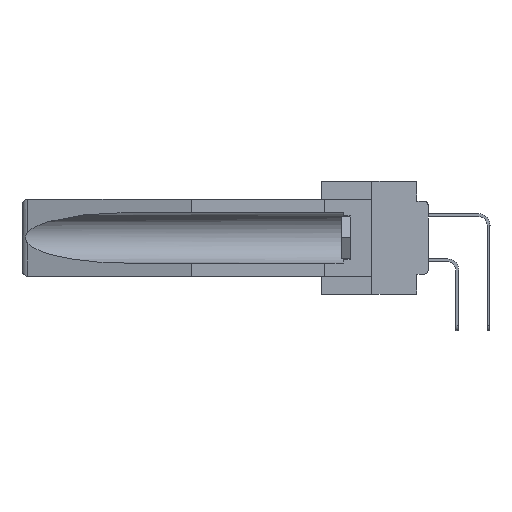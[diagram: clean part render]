
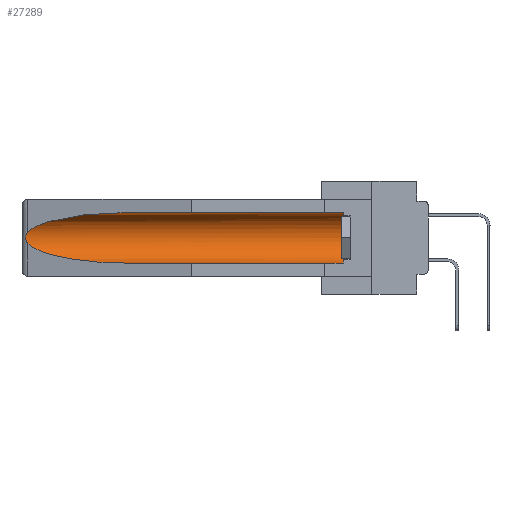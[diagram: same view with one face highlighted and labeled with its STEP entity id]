
A CAD part, left-side view. The second image highlights one B-rep face of the part: STEP entity #27289.
In plain terms, the highlighted cylindrical face has radius 2.857 mm (diameter 5.715 mm), a partial arc.
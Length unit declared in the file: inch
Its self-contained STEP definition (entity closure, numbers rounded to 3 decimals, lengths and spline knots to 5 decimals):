
#214 = VECTOR ( 'NONE', #16358, 39.37008 ) ;
#220 = EDGE_CURVE ( 'NONE', #14989, #16163, #27075, .T. ) ;
#622 = LINE ( 'NONE', #17591, #22958 ) ;
#1041 = CARTESIAN_POINT ( 'NONE',  ( 0.2675, 1.53308, -0.17534 ) ) ;
#2918 = VERTEX_POINT ( 'NONE', #24514 ) ;
#2966 = CARTESIAN_POINT ( 'NONE',  ( 0.25451, 1.48313, -0.24835 ) ) ;
#3231 = EDGE_LOOP ( 'NONE', ( #13772, #20489, #29603, #16007, #25801, #6944 ) ) ;
#3572 = CARTESIAN_POINT ( 'NONE',  ( 0.26537, 1.52718, -0.14972 ) ) ;
#3773 = CARTESIAN_POINT ( 'NONE',  ( 0.21114, 1.30732, -0.059 ) ) ;
#5889 = CARTESIAN_POINT ( 'NONE',  ( 0.26537, 1.52718, -0.19328 ) ) ;
#6092 = CARTESIAN_POINT ( 'NONE',  ( 0.2673, 1.53269, -0.17917 ) ) ;
#6944 = ORIENTED_EDGE ( 'NONE', *, *, #20232, .T. ) ;
#7067 = CARTESIAN_POINT ( 'NONE',  ( 0.155, -0.30754, -0.1715 ) ) ;
#7306 = DIRECTION ( 'NONE',  ( 0., 0., 1. ) ) ;
#7380 = DIRECTION ( 'NONE',  ( 0., 1., 0. ) ) ;
#8612 = VERTEX_POINT ( 'NONE', #22901 ) ;
#8885 = EDGE_CURVE ( 'NONE', #26330, #2918, #29092, .T. ) ;
#10323 = CARTESIAN_POINT ( 'NONE',  ( 0.26537, 1.52718, -0.14972 ) ) ;
#11713 = EDGE_CURVE ( 'NONE', #14989, #24614, #28343, .T. ) ;
#12687 = CARTESIAN_POINT ( 'NONE',  ( 0.155, 0.126, -0.284 ) ) ;
#13161 = CARTESIAN_POINT ( 'NONE',  ( 0.26654, 1.53092, -0.15636 ) ) ;
#13772 = ORIENTED_EDGE ( 'NONE', *, *, #15866, .T. ) ;
#13786 = CYLINDRICAL_SURFACE ( 'NONE', #28891, 0.1125 ) ;
#14078 = CARTESIAN_POINT ( 'NONE',  ( 0.155, 1.07973, -0.284 ) ) ;
#14661 = CARTESIAN_POINT ( 'NONE',  ( 0.155, 0.126, -0.1715 ) ) ;
#14989 = VERTEX_POINT ( 'NONE', #12687 ) ;
#15505 = CARTESIAN_POINT ( 'NONE',  ( 0.26537, 1.52718, -0.19328 ) ) ;
#15866 = EDGE_CURVE ( 'NONE', #8612, #26330, #23485, .T. ) ;
#16007 = ORIENTED_EDGE ( 'NONE', *, *, #220, .F. ) ;
#16163 = VERTEX_POINT ( 'NONE', #14078 ) ;
#16358 = DIRECTION ( 'NONE',  ( 0., 1., 0. ) ) ;
#16474 = CARTESIAN_POINT ( 'NONE',  ( 0.155, -0.30754, -0.284 ) ) ;
#16822 = DIRECTION ( 'NONE',  ( 0., -1., 0. ) ) ;
#17359 = CARTESIAN_POINT ( 'NONE',  ( 0.155, 1.07973, -0.284 ) ) ;
#17591 = CARTESIAN_POINT ( 'NONE',  ( 0.155, -0.30754, -0.059 ) ) ;
#17766 = CARTESIAN_POINT ( 'NONE',  ( 0.2673, 1.5327, -0.16383 ) ) ;
#17868 = CARTESIAN_POINT ( 'NONE',  ( 0.26655, 1.53094, -0.18657 ) ) ;
#18258 = CARTESIAN_POINT ( 'NONE',  ( 0.155, 0.126, -0.059 ) ) ;
#19763 = CARTESIAN_POINT ( 'NONE',  ( 0.26537, 1.52718, -0.14972 ) ) ;
#19903 = FACE_OUTER_BOUND ( 'NONE', #3231, .T. ) ;
#20130 = DIRECTION ( 'NONE',  ( 0., 1., 0. ) ) ;
#20232 = EDGE_CURVE ( 'NONE', #24614, #8612, #622, .T. ) ;
#20401 = CARTESIAN_POINT ( 'NONE',  ( 0.26597, 1.52961, -0.15275 ) ) ;
#20489 = ORIENTED_EDGE ( 'NONE', *, *, #8885, .T. ) ;
#20605 = CARTESIAN_POINT ( 'NONE',  ( 0.2675, 1.53308, -0.16763 ) ) ;
#20769 =( BOUNDED_CURVE ( )  B_SPLINE_CURVE ( 3, ( #15505, #2966, #22012, #17359 ),
 .UNSPECIFIED., .F., .F. ) 
 B_SPLINE_CURVE_WITH_KNOTS ( ( 4, 4 ),
 ( 0.1948, 1.5708 ),
 .UNSPECIFIED. ) 
 CURVE ( )  GEOMETRIC_REPRESENTATION_ITEM ( )  RATIONAL_B_SPLINE_CURVE ( ( 1., 0.848, 0.848, 1. ) ) 
 REPRESENTATION_ITEM ( '' )  );
#21565 = DIRECTION ( 'NONE',  ( 0., 0., 1. ) ) ;
#21851 = AXIS2_PLACEMENT_3D ( 'NONE', #14661, #16822, #7306 ) ;
#22012 = CARTESIAN_POINT ( 'NONE',  ( 0.21114, 1.30732, -0.284 ) ) ;
#22901 = CARTESIAN_POINT ( 'NONE',  ( 0.155, 1.07973, -0.059 ) ) ;
#22958 = VECTOR ( 'NONE', #20130, 39.37008 ) ;
#23035 = CARTESIAN_POINT ( 'NONE',  ( 0.26597, 1.5296, -0.19026 ) ) ;
#23485 =( BOUNDED_CURVE ( )  B_SPLINE_CURVE ( 3, ( #25539, #3773, #27874, #3572 ),
 .UNSPECIFIED., .F., .T. ) 
 B_SPLINE_CURVE_WITH_KNOTS ( ( 4, 4 ),
 ( 4.71239, 6.08839 ),
 .UNSPECIFIED. ) 
 CURVE ( )  GEOMETRIC_REPRESENTATION_ITEM ( )  RATIONAL_B_SPLINE_CURVE ( ( 1., 0.848, 0.848, 1. ) ) 
 REPRESENTATION_ITEM ( '' )  );
#24514 = CARTESIAN_POINT ( 'NONE',  ( 0.26537, 1.52718, -0.19328 ) ) ;
#24614 = VERTEX_POINT ( 'NONE', #18258 ) ;
#25539 = CARTESIAN_POINT ( 'NONE',  ( 0.155, 1.07973, -0.059 ) ) ;
#25801 = ORIENTED_EDGE ( 'NONE', *, *, #11713, .T. ) ;
#26330 = VERTEX_POINT ( 'NONE', #19763 ) ;
#27075 = LINE ( 'NONE', #16474, #214 ) ;
#27289 = ADVANCED_FACE ( 'NONE', ( #19903 ), #13786, .F. ) ;
#27874 = CARTESIAN_POINT ( 'NONE',  ( 0.25451, 1.48313, -0.09465 ) ) ;
#28343 = CIRCLE ( 'NONE', #21851, 0.1125 ) ;
#28358 = EDGE_CURVE ( 'NONE', #2918, #16163, #20769, .T. ) ;
#28891 = AXIS2_PLACEMENT_3D ( 'NONE', #7067, #7380, #21565 ) ;
#29092 = B_SPLINE_CURVE_WITH_KNOTS ( 'NONE', 3,
 ( #10323, #20401, #13161, #17766, #20605, #1041, #6092, #17868, #23035, #5889 ),
 .UNSPECIFIED., .F., .F.,
 ( 4, 2, 2, 2, 4 ),
 ( 0., 0.00029, 0.00058, 0.00087, 0.00117 ),
 .UNSPECIFIED. ) ;
#29603 = ORIENTED_EDGE ( 'NONE', *, *, #28358, .T. ) ;
